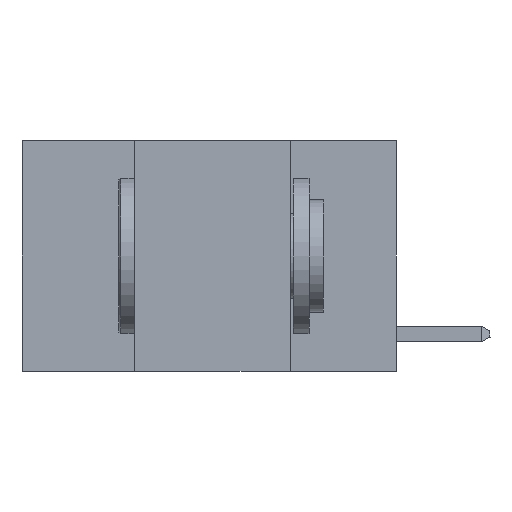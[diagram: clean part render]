
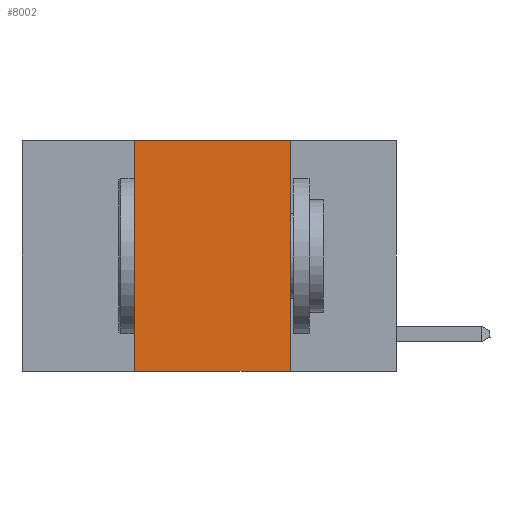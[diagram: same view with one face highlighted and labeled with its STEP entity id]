
A CAD part, left-side view. The second image highlights one B-rep face of the part: STEP entity #8002.
In plain terms, the highlighted planar face has unit normal (-1, 0, 0).
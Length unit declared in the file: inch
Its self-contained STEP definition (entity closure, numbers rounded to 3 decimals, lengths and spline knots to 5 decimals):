
#109 = LINE ( 'NONE', #1127, #7996 ) ;
#188 = CARTESIAN_POINT ( 'NONE',  ( 0., 0.17, 0. ) ) ;
#482 = LINE ( 'NONE', #6647, #2888 ) ;
#646 = DIRECTION ( 'NONE',  ( 0., -1., 0. ) ) ;
#937 = ORIENTED_EDGE ( 'NONE', *, *, #2410, .T. ) ;
#1127 = CARTESIAN_POINT ( 'NONE',  ( 0., 0.6, 0. ) ) ;
#1579 = VECTOR ( 'NONE', #9458, 39.37008 ) ;
#1790 = FACE_OUTER_BOUND ( 'NONE', #3047, .T. ) ;
#2088 = DIRECTION ( 'NONE',  ( 1., 0., 0. ) ) ;
#2410 = EDGE_CURVE ( 'NONE', #6836, #5551, #482, .T. ) ;
#2522 = AXIS2_PLACEMENT_3D ( 'NONE', #6173, #2088, #9284 ) ;
#2839 = VECTOR ( 'NONE', #10518, 39.37008 ) ;
#2888 = VECTOR ( 'NONE', #6539, 39.37008 ) ;
#3047 = EDGE_LOOP ( 'NONE', ( #9156, #8183, #8490, #937 ) ) ;
#3118 = EDGE_CURVE ( 'NONE', #6836, #9772, #4346, .T. ) ;
#3199 = CARTESIAN_POINT ( 'NONE',  ( 0., 0.42, -0.37 ) ) ;
#4181 = EDGE_CURVE ( 'NONE', #9772, #7496, #109, .T. ) ;
#4346 = LINE ( 'NONE', #10229, #1579 ) ;
#4363 = CARTESIAN_POINT ( 'NONE',  ( 0., 0.17, 0. ) ) ;
#5166 = EDGE_CURVE ( 'NONE', #7496, #5551, #11063, .T. ) ;
#5551 = VERTEX_POINT ( 'NONE', #11150 ) ;
#5969 = CARTESIAN_POINT ( 'NONE',  ( 0., 0.42, 0. ) ) ;
#6173 = CARTESIAN_POINT ( 'NONE',  ( 0., 0.6, 0. ) ) ;
#6539 = DIRECTION ( 'NONE',  ( 0., -1., 0. ) ) ;
#6647 = CARTESIAN_POINT ( 'NONE',  ( 0., 0.6, -0.37 ) ) ;
#6836 = VERTEX_POINT ( 'NONE', #3199 ) ;
#7496 = VERTEX_POINT ( 'NONE', #188 ) ;
#7996 = VECTOR ( 'NONE', #646, 39.37008 ) ;
#8002 = ADVANCED_FACE ( 'NONE', ( #1790 ), #12279, .F. ) ;
#8183 = ORIENTED_EDGE ( 'NONE', *, *, #4181, .F. ) ;
#8490 = ORIENTED_EDGE ( 'NONE', *, *, #3118, .F. ) ;
#9156 = ORIENTED_EDGE ( 'NONE', *, *, #5166, .F. ) ;
#9284 = DIRECTION ( 'NONE',  ( 0., 0., -1. ) ) ;
#9458 = DIRECTION ( 'NONE',  ( 0., 0., 1. ) ) ;
#9772 = VERTEX_POINT ( 'NONE', #5969 ) ;
#10229 = CARTESIAN_POINT ( 'NONE',  ( 0., 0.42, 0. ) ) ;
#10518 = DIRECTION ( 'NONE',  ( 0., 0., -1. ) ) ;
#11063 = LINE ( 'NONE', #4363, #2839 ) ;
#11150 = CARTESIAN_POINT ( 'NONE',  ( 0., 0.17, -0.37 ) ) ;
#12279 = PLANE ( 'NONE',  #2522 ) ;
